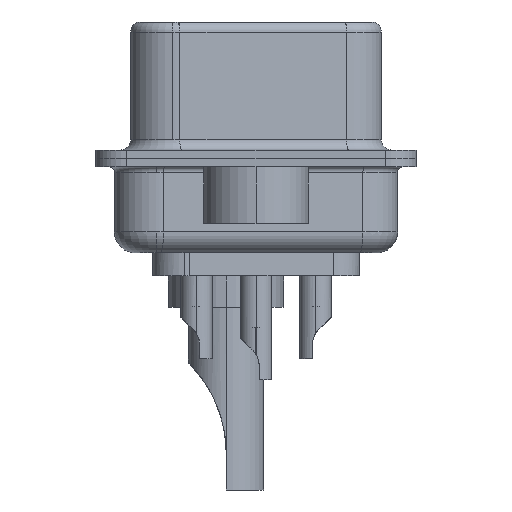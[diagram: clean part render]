
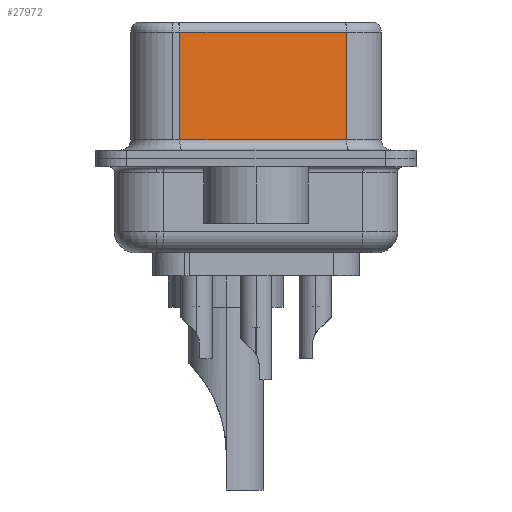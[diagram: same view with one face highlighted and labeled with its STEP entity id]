
A CAD part, left-side view. The second image highlights one B-rep face of the part: STEP entity #27972.
In plain terms, the highlighted planar face has unit normal (-0.985, -0.174, 0).
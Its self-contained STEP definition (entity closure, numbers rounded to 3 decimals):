
#1198 = CARTESIAN_POINT ( 'NONE',  ( 5.132, -4.322, 6.02 ) ) ;
#1273 = LINE ( 'NONE', #8405, #1616 ) ;
#1440 = EDGE_CURVE ( 'NONE', #21165, #23919, #19886, .T. ) ;
#1616 = VECTOR ( 'NONE', #14917, 1000. ) ;
#2355 = VECTOR ( 'NONE', #24290, 1000. ) ;
#2656 = CARTESIAN_POINT ( 'NONE',  ( 5.132, -4.322, 0.9 ) ) ;
#2807 = DIRECTION ( 'NONE',  ( -0.174, 0.985, 0. ) ) ;
#3129 = CARTESIAN_POINT ( 'NONE',  ( 5.132, -4.322, 6.52 ) ) ;
#3770 = EDGE_CURVE ( 'NONE', #21165, #22174, #13964, .T. ) ;
#3922 = CARTESIAN_POINT ( 'NONE',  ( 3.73, 3.628, 0.9 ) ) ;
#7267 = CARTESIAN_POINT ( 'NONE',  ( 5.132, -4.322, 6.02 ) ) ;
#7984 = LINE ( 'NONE', #12912, #21781 ) ;
#8405 = CARTESIAN_POINT ( 'NONE',  ( 3.73, 3.628, 6.52 ) ) ;
#9863 = DIRECTION ( 'NONE',  ( 0.985, 0.174, 0. ) ) ;
#11808 = ORIENTED_EDGE ( 'NONE', *, *, #28897, .T. ) ;
#12308 = CARTESIAN_POINT ( 'NONE',  ( 5.132, -4.322, 6.52 ) ) ;
#12912 = CARTESIAN_POINT ( 'NONE',  ( 5.132, -4.322, 0.9 ) ) ;
#13964 = LINE ( 'NONE', #3129, #26323 ) ;
#14917 = DIRECTION ( 'NONE',  ( 0., 0., -1. ) ) ;
#15266 = DIRECTION ( 'NONE',  ( 0.174, -0.985, 0. ) ) ;
#17013 = EDGE_LOOP ( 'NONE', ( #27910, #19821, #11808, #28815 ) ) ;
#19821 = ORIENTED_EDGE ( 'NONE', *, *, #1440, .T. ) ;
#19886 = LINE ( 'NONE', #1198, #2355 ) ;
#21165 = VERTEX_POINT ( 'NONE', #7267 ) ;
#21306 = FACE_OUTER_BOUND ( 'NONE', #17013, .T. ) ;
#21752 = DIRECTION ( 'NONE',  ( 0., 0., -1. ) ) ;
#21781 = VECTOR ( 'NONE', #15266, 1000. ) ;
#22174 = VERTEX_POINT ( 'NONE', #2656 ) ;
#23919 = VERTEX_POINT ( 'NONE', #24311 ) ;
#24290 = DIRECTION ( 'NONE',  ( -0.174, 0.985, 0. ) ) ;
#24311 = CARTESIAN_POINT ( 'NONE',  ( 3.73, 3.628, 6.02 ) ) ;
#25759 = AXIS2_PLACEMENT_3D ( 'NONE', #12308, #9863, #2807 ) ;
#26030 = EDGE_CURVE ( 'NONE', #28298, #22174, #7984, .T. ) ;
#26323 = VECTOR ( 'NONE', #21752, 1000. ) ;
#27910 = ORIENTED_EDGE ( 'NONE', *, *, #3770, .F. ) ;
#27972 = ADVANCED_FACE ( 'NONE', ( #21306 ), #28666, .F. ) ;
#28298 = VERTEX_POINT ( 'NONE', #3922 ) ;
#28666 = PLANE ( 'NONE',  #25759 ) ;
#28815 = ORIENTED_EDGE ( 'NONE', *, *, #26030, .T. ) ;
#28897 = EDGE_CURVE ( 'NONE', #23919, #28298, #1273, .T. ) ;
